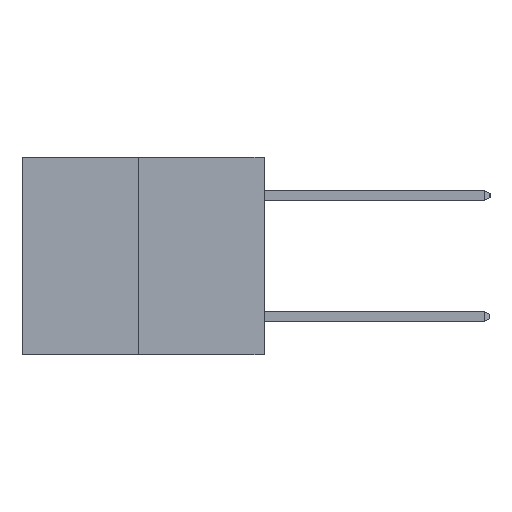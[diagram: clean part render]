
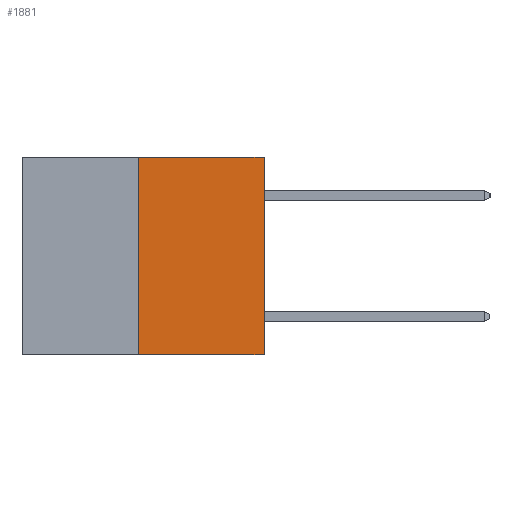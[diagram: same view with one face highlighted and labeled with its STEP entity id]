
A CAD part, left-side view. The second image highlights one B-rep face of the part: STEP entity #1881.
In plain terms, the highlighted planar face has unit normal (-1, 0, 0).
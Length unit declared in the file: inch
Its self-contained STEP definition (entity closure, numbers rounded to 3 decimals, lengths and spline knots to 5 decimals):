
#476 = CARTESIAN_POINT ( 'NONE',  ( 0., 0., 0. ) ) ;
#886 = DIRECTION ( 'NONE',  ( 0., -1., 0. ) ) ;
#1187 = VERTEX_POINT ( 'NONE', #1373 ) ;
#1188 = DIRECTION ( 'NONE',  ( 0., 0., -1. ) ) ;
#1308 = EDGE_CURVE ( 'NONE', #1187, #4813, #8462, .T. ) ;
#1373 = CARTESIAN_POINT ( 'NONE',  ( 0., 0.312, -0.49 ) ) ;
#1683 = DIRECTION ( 'NONE',  ( 0., -1., 0. ) ) ;
#1859 = EDGE_CURVE ( 'NONE', #1187, #6755, #4204, .T. ) ;
#1881 = ADVANCED_FACE ( 'NONE', ( #8931 ), #2247, .F. ) ;
#2247 = PLANE ( 'NONE',  #11796 ) ;
#2326 = CARTESIAN_POINT ( 'NONE',  ( 0., 0.312, -0.49 ) ) ;
#3169 = VECTOR ( 'NONE', #886, 39.37008 ) ;
#3282 = ORIENTED_EDGE ( 'NONE', *, *, #11084, .F. ) ;
#3644 = CARTESIAN_POINT ( 'NONE',  ( 0., 0.6, -0.49 ) ) ;
#3763 = EDGE_CURVE ( 'NONE', #4813, #4544, #9141, .T. ) ;
#4204 = LINE ( 'NONE', #2326, #12084 ) ;
#4544 = VERTEX_POINT ( 'NONE', #476 ) ;
#4813 = VERTEX_POINT ( 'NONE', #9727 ) ;
#4821 = VECTOR ( 'NONE', #13107, 39.37008 ) ;
#5318 = DIRECTION ( 'NONE',  ( 1., 0., 0. ) ) ;
#6755 = VERTEX_POINT ( 'NONE', #11691 ) ;
#7365 = CARTESIAN_POINT ( 'NONE',  ( 0., 0.6, 0. ) ) ;
#8132 = LINE ( 'NONE', #10108, #3169 ) ;
#8462 = LINE ( 'NONE', #3644, #10237 ) ;
#8931 = FACE_OUTER_BOUND ( 'NONE', #12528, .T. ) ;
#9141 = LINE ( 'NONE', #12032, #4821 ) ;
#9727 = CARTESIAN_POINT ( 'NONE',  ( 0., 0., -0.49 ) ) ;
#10108 = CARTESIAN_POINT ( 'NONE',  ( 0., 0.6, 0. ) ) ;
#10237 = VECTOR ( 'NONE', #1683, 39.37008 ) ;
#10482 = DIRECTION ( 'NONE',  ( 0., 0., 1. ) ) ;
#11084 = EDGE_CURVE ( 'NONE', #6755, #4544, #8132, .T. ) ;
#11481 = ORIENTED_EDGE ( 'NONE', *, *, #3763, .T. ) ;
#11691 = CARTESIAN_POINT ( 'NONE',  ( 0., 0.312, 0. ) ) ;
#11796 = AXIS2_PLACEMENT_3D ( 'NONE', #7365, #5318, #1188 ) ;
#11923 = ORIENTED_EDGE ( 'NONE', *, *, #1859, .F. ) ;
#12032 = CARTESIAN_POINT ( 'NONE',  ( 0., 0., 0. ) ) ;
#12084 = VECTOR ( 'NONE', #10482, 39.37008 ) ;
#12528 = EDGE_LOOP ( 'NONE', ( #11923, #12837, #11481, #3282 ) ) ;
#12837 = ORIENTED_EDGE ( 'NONE', *, *, #1308, .T. ) ;
#13107 = DIRECTION ( 'NONE',  ( 0., 0., 1. ) ) ;
